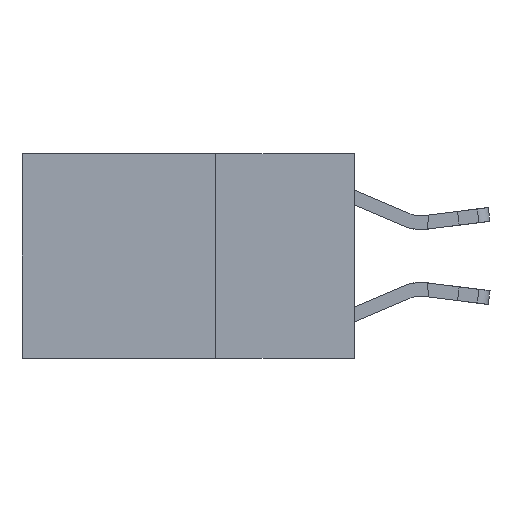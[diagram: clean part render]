
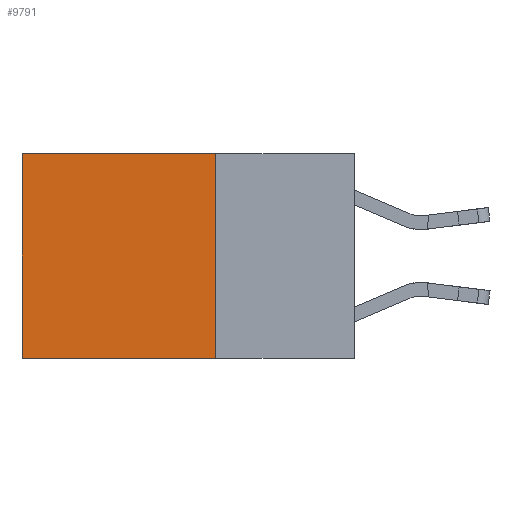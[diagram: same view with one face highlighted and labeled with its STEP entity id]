
A CAD part, left-side view. The second image highlights one B-rep face of the part: STEP entity #9791.
In plain terms, the highlighted planar face has unit normal (-1, 0, 0).
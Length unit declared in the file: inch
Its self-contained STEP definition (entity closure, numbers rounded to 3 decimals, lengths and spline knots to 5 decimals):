
#117 = LINE ( 'NONE', #10899, #17835 ) ;
#134 = DIRECTION ( 'NONE',  ( 0., 0., -1. ) ) ;
#529 = ORIENTED_EDGE ( 'NONE', *, *, #3588, .F. ) ;
#1334 = LINE ( 'NONE', #4033, #4697 ) ;
#1839 = VECTOR ( 'NONE', #10689, 39.37008 ) ;
#1986 = CARTESIAN_POINT ( 'NONE',  ( 0.2625, 0.25, 0. ) ) ;
#3265 = VERTEX_POINT ( 'NONE', #8852 ) ;
#3588 = EDGE_CURVE ( 'NONE', #6643, #7021, #13043, .T. ) ;
#3904 = ORIENTED_EDGE ( 'NONE', *, *, #13100, .T. ) ;
#4033 = CARTESIAN_POINT ( 'NONE',  ( 0.2625, 0.25, -0.37 ) ) ;
#4288 = EDGE_LOOP ( 'NONE', ( #17722, #13605, #529, #3904 ) ) ;
#4371 = EDGE_CURVE ( 'NONE', #3265, #16570, #117, .T. ) ;
#4697 = VECTOR ( 'NONE', #14888, 39.37008 ) ;
#4771 = AXIS2_PLACEMENT_3D ( 'NONE', #15416, #19783, #134 ) ;
#6358 = CARTESIAN_POINT ( 'NONE',  ( 0.2625, 0.25, 0. ) ) ;
#6643 = VERTEX_POINT ( 'NONE', #1986 ) ;
#7021 = VERTEX_POINT ( 'NONE', #7901 ) ;
#7322 = VECTOR ( 'NONE', #15944, 39.37008 ) ;
#7901 = CARTESIAN_POINT ( 'NONE',  ( 0.2625, 0.25, -0.37 ) ) ;
#7977 = DIRECTION ( 'NONE',  ( 0., 0., -1. ) ) ;
#8852 = CARTESIAN_POINT ( 'NONE',  ( 0.2625, 0.6, 0. ) ) ;
#9791 = ADVANCED_FACE ( 'NONE', ( #16925 ), #16622, .F. ) ;
#10689 = DIRECTION ( 'NONE',  ( 0., 1., 0. ) ) ;
#10785 = LINE ( 'NONE', #6358, #1839 ) ;
#10899 = CARTESIAN_POINT ( 'NONE',  ( 0.2625, 0.6, 0. ) ) ;
#12882 = EDGE_CURVE ( 'NONE', #7021, #16570, #1334, .T. ) ;
#12890 = CARTESIAN_POINT ( 'NONE',  ( 0.2625, 0.6, -0.37 ) ) ;
#13043 = LINE ( 'NONE', #19022, #7322 ) ;
#13100 = EDGE_CURVE ( 'NONE', #6643, #3265, #10785, .T. ) ;
#13605 = ORIENTED_EDGE ( 'NONE', *, *, #12882, .F. ) ;
#14888 = DIRECTION ( 'NONE',  ( 0., 1., 0. ) ) ;
#15416 = CARTESIAN_POINT ( 'NONE',  ( 0.2625, 0.25, 0. ) ) ;
#15944 = DIRECTION ( 'NONE',  ( 0., 0., -1. ) ) ;
#16570 = VERTEX_POINT ( 'NONE', #12890 ) ;
#16622 = PLANE ( 'NONE',  #4771 ) ;
#16925 = FACE_OUTER_BOUND ( 'NONE', #4288, .T. ) ;
#17722 = ORIENTED_EDGE ( 'NONE', *, *, #4371, .T. ) ;
#17835 = VECTOR ( 'NONE', #7977, 39.37008 ) ;
#19022 = CARTESIAN_POINT ( 'NONE',  ( 0.2625, 0.25, 0. ) ) ;
#19783 = DIRECTION ( 'NONE',  ( 1., 0., 0. ) ) ;
